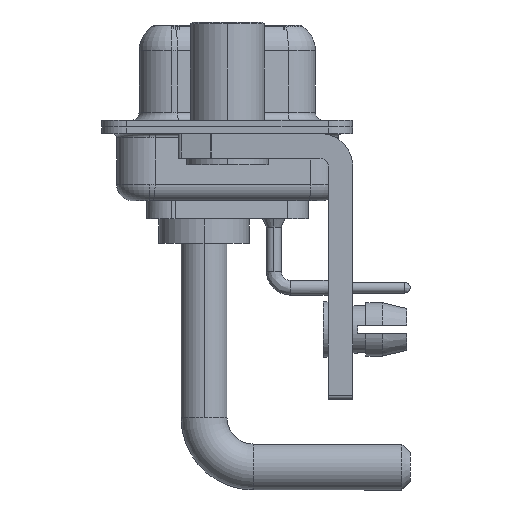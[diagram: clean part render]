
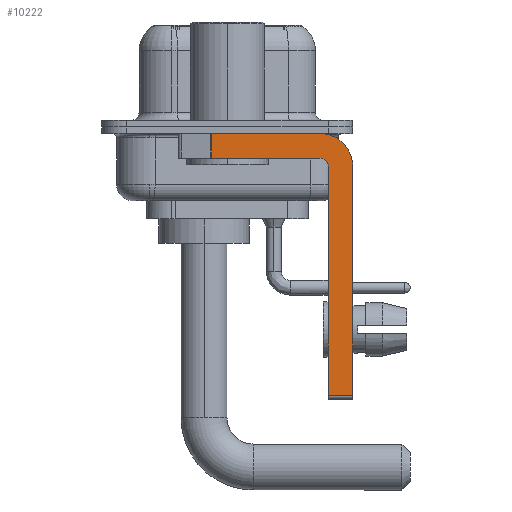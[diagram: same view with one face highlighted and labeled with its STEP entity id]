
A CAD part, left-side view. The second image highlights one B-rep face of the part: STEP entity #10222.
In plain terms, the highlighted planar face has unit normal (-1, 0, 0).
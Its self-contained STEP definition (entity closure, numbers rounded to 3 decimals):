
#35 = LINE ( 'NONE', #1894, #21433 ) ;
#107 = ORIENTED_EDGE ( 'NONE', *, *, #10855, .F. ) ;
#853 = FACE_OUTER_BOUND ( 'NONE', #14779, .T. ) ;
#1894 = CARTESIAN_POINT ( 'NONE',  ( -2.9, 0.978, -1.9 ) ) ;
#2065 = ORIENTED_EDGE ( 'NONE', *, *, #6214, .T. ) ;
#2096 = CARTESIAN_POINT ( 'NONE',  ( -2.9, -6.15, -2.4 ) ) ;
#2210 = DIRECTION ( 'NONE',  ( 0., 0., 1. ) ) ;
#2249 = DIRECTION ( 'NONE',  ( 0., 0., 1. ) ) ;
#2458 = DIRECTION ( 'NONE',  ( 1., 0., 0. ) ) ;
#2673 = DIRECTION ( 'NONE',  ( 0., -1., 0. ) ) ;
#2784 = VERTEX_POINT ( 'NONE', #23856 ) ;
#2815 = VERTEX_POINT ( 'NONE', #12477 ) ;
#2976 = DIRECTION ( 'NONE',  ( 1., 0., 0. ) ) ;
#3364 = VECTOR ( 'NONE', #12074, 1000. ) ;
#3555 = EDGE_CURVE ( 'NONE', #2784, #20598, #12210, .T. ) ;
#3576 = CIRCLE ( 'NONE', #23973, 2. ) ;
#3966 = DIRECTION ( 'NONE',  ( 0., 1., 0. ) ) ;
#4256 = CARTESIAN_POINT ( 'NONE',  ( -2.9, -5.65, -2.4 ) ) ;
#4347 = AXIS2_PLACEMENT_3D ( 'NONE', #14507, #2976, #18016 ) ;
#4530 = DIRECTION ( 'NONE',  ( 0., 0., -1. ) ) ;
#4978 = ORIENTED_EDGE ( 'NONE', *, *, #7085, .F. ) ;
#5195 = VECTOR ( 'NONE', #3966, 1000. ) ;
#5398 = VERTEX_POINT ( 'NONE', #7257 ) ;
#5753 = ORIENTED_EDGE ( 'NONE', *, *, #3555, .F. ) ;
#6115 = VERTEX_POINT ( 'NONE', #19978 ) ;
#6214 = EDGE_CURVE ( 'NONE', #2784, #2815, #35, .T. ) ;
#6528 = CARTESIAN_POINT ( 'NONE',  ( -2.9, -5.65, -16.35 ) ) ;
#6937 = EDGE_CURVE ( 'NONE', #18477, #6115, #24179, .T. ) ;
#7085 = EDGE_CURVE ( 'NONE', #15940, #18477, #12120, .T. ) ;
#7257 = CARTESIAN_POINT ( 'NONE',  ( -2.9, -7.65, -2.4 ) ) ;
#7455 = LINE ( 'NONE', #7711, #5195 ) ;
#7711 = CARTESIAN_POINT ( 'NONE',  ( -2.9, -5.65, -1.9 ) ) ;
#8365 = ORIENTED_EDGE ( 'NONE', *, *, #19121, .T. ) ;
#8607 = PLANE ( 'NONE',  #4347 ) ;
#8949 = VECTOR ( 'NONE', #4530, 1000. ) ;
#9085 = ORIENTED_EDGE ( 'NONE', *, *, #17304, .F. ) ;
#10222 = ADVANCED_FACE ( 'NONE', ( #853 ), #8607, .F. ) ;
#10540 = CARTESIAN_POINT ( 'NONE',  ( -2.9, -6.15, -16.35 ) ) ;
#10855 = EDGE_CURVE ( 'NONE', #20598, #5398, #3576, .T. ) ;
#11203 = EDGE_CURVE ( 'NONE', #6115, #2815, #7455, .T. ) ;
#11990 = CARTESIAN_POINT ( 'NONE',  ( -2.9, -5.65, -2.4 ) ) ;
#12074 = DIRECTION ( 'NONE',  ( 0., -1., 0. ) ) ;
#12120 = LINE ( 'NONE', #13990, #14210 ) ;
#12210 = LINE ( 'NONE', #19817, #13967 ) ;
#12211 = AXIS2_PLACEMENT_3D ( 'NONE', #4256, #19397, #2249 ) ;
#12477 = CARTESIAN_POINT ( 'NONE',  ( -2.9, 0.978, -1.9 ) ) ;
#13967 = VECTOR ( 'NONE', #2673, 1000. ) ;
#13990 = CARTESIAN_POINT ( 'NONE',  ( -2.9, -6.15, -16.6 ) ) ;
#14061 = LINE ( 'NONE', #21685, #8949 ) ;
#14210 = VECTOR ( 'NONE', #2210, 1000. ) ;
#14507 = CARTESIAN_POINT ( 'NONE',  ( -2.9, -5.65, -2.4 ) ) ;
#14593 = ORIENTED_EDGE ( 'NONE', *, *, #11203, .F. ) ;
#14610 = DIRECTION ( 'NONE',  ( 0., 0., -1. ) ) ;
#14779 = EDGE_LOOP ( 'NONE', ( #5753, #2065, #14593, #22474, #4978, #8365, #9085, #107 ) ) ;
#14957 = CARTESIAN_POINT ( 'NONE',  ( -2.9, -7.65, -16.35 ) ) ;
#15940 = VERTEX_POINT ( 'NONE', #10540 ) ;
#17304 = EDGE_CURVE ( 'NONE', #5398, #18854, #14061, .T. ) ;
#17859 = DIRECTION ( 'NONE',  ( 0., 0., -1. ) ) ;
#18016 = DIRECTION ( 'NONE',  ( 0., 0., -1. ) ) ;
#18477 = VERTEX_POINT ( 'NONE', #2096 ) ;
#18854 = VERTEX_POINT ( 'NONE', #14957 ) ;
#19121 = EDGE_CURVE ( 'NONE', #15940, #18854, #23692, .T. ) ;
#19397 = DIRECTION ( 'NONE',  ( -1., 0., 0. ) ) ;
#19653 = CARTESIAN_POINT ( 'NONE',  ( -2.9, -5.65, -0.4 ) ) ;
#19817 = CARTESIAN_POINT ( 'NONE',  ( -2.9, 3., -0.4 ) ) ;
#19978 = CARTESIAN_POINT ( 'NONE',  ( -2.9, -5.65, -1.9 ) ) ;
#20598 = VERTEX_POINT ( 'NONE', #19653 ) ;
#21433 = VECTOR ( 'NONE', #14610, 1000. ) ;
#21685 = CARTESIAN_POINT ( 'NONE',  ( -2.9, -7.65, -2.4 ) ) ;
#22474 = ORIENTED_EDGE ( 'NONE', *, *, #6937, .F. ) ;
#23692 = LINE ( 'NONE', #6528, #3364 ) ;
#23856 = CARTESIAN_POINT ( 'NONE',  ( -2.9, 0.978, -0.4 ) ) ;
#23973 = AXIS2_PLACEMENT_3D ( 'NONE', #11990, #2458, #17859 ) ;
#24179 = CIRCLE ( 'NONE', #12211, 0.5 ) ;
